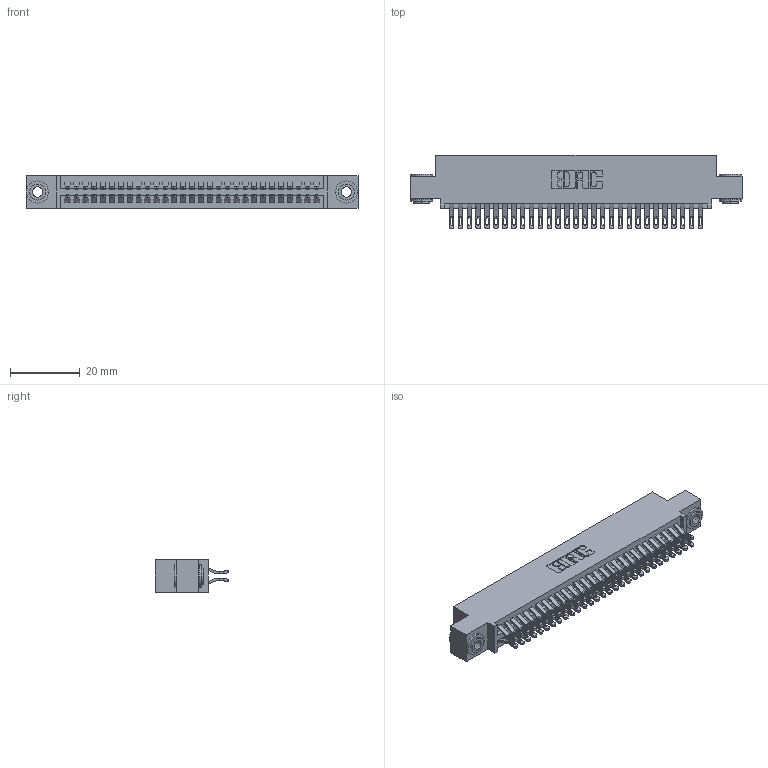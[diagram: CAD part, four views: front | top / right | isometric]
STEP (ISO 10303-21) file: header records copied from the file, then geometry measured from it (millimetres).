
FILE_DESCRIPTION (( 'STEP AP203' ), '1' );
FILE_NAME ('345-058-555-503.STEP', '2019-10-30T05:54:36', ( '' ), ( '' ), 'SwSTEP 2.0', 'SolidWorks 2016', '' );
FILE_SCHEMA (( 'CONFIG_CONTROL_DESIGN' ));
Length unit declared in the file: inch
Products named in the file (4): 345-292-001_555 Tail; 345-058-555-503; 345 Part_0.110 Offset - 0.156 Dia-TH; 345-250-002_345-250-002-102
Assembly tree (61 placements, depth 2):
  345-058-555-503
    345 Part_0.110 Offset - 0.156 Dia-TH
    345-292-001_555 Tail  x58
    345-250-002_345-250-002-102  x2
Bounding box: 94.87 x 21.13 x 9.4 mm (x, y, z)
Volume: 9209.3 mm3; surface area: 14243.9 mm2
Topology: 61 solids, 61 shells, 3416 faces, 10695 edges, 7126 vertices
Faces by surface type: plane 1892, cylinder 1516, cone 8
Entity records: 25612 total; most frequent: CARTESIAN_POINT 4317, ORIENTED_EDGE 4214, DIRECTION 3821, EDGE_CURVE 2107, LINE 1815, VECTOR 1815, VERTEX_POINT 1402, AXIS2_PLACEMENT_3D 1003
